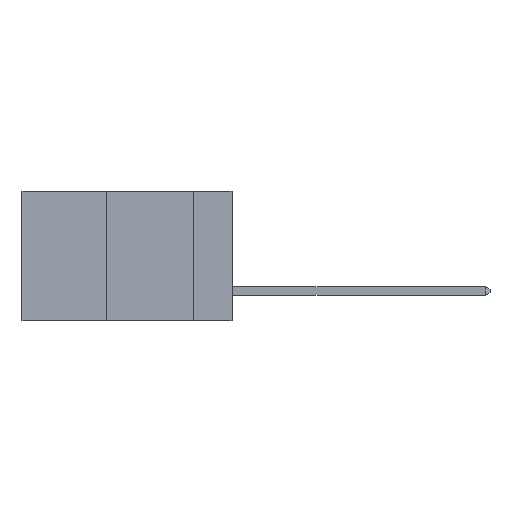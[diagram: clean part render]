
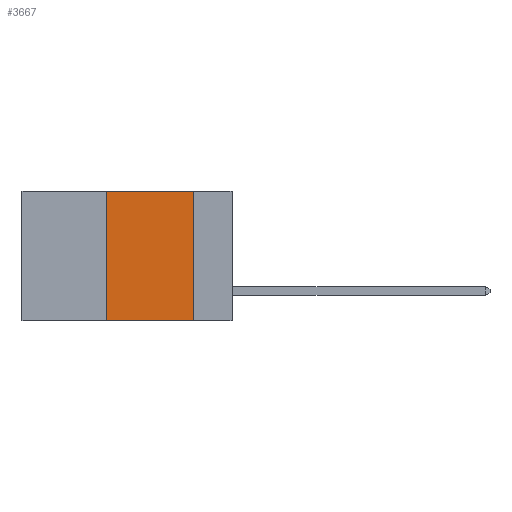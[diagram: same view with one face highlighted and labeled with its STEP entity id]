
A CAD part, left-side view. The second image highlights one B-rep face of the part: STEP entity #3667.
In plain terms, the highlighted planar face has unit normal (-1, 0, 0).
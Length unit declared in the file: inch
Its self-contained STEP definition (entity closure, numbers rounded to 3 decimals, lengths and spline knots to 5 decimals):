
#189 = EDGE_CURVE ( 'NONE', #11978, #1055, #10792, .T. ) ;
#576 = ORIENTED_EDGE ( 'NONE', *, *, #189, .F. ) ;
#738 = CARTESIAN_POINT ( 'NONE',  ( 0., 0.36, 0. ) ) ;
#850 = CARTESIAN_POINT ( 'NONE',  ( 0., 0.6, -0.37 ) ) ;
#1055 = VERTEX_POINT ( 'NONE', #12014 ) ;
#1774 = AXIS2_PLACEMENT_3D ( 'NONE', #11319, #6439, #12218 ) ;
#1845 = DIRECTION ( 'NONE',  ( 0., -1., 0. ) ) ;
#2360 = ORIENTED_EDGE ( 'NONE', *, *, #4052, .F. ) ;
#2379 = CARTESIAN_POINT ( 'NONE',  ( 0., 0.36, -0.37 ) ) ;
#2485 = VERTEX_POINT ( 'NONE', #2379 ) ;
#2753 = CARTESIAN_POINT ( 'NONE',  ( 0., 0.11, 0. ) ) ;
#3005 = DIRECTION ( 'NONE',  ( 0., -1., 0. ) ) ;
#3048 = CARTESIAN_POINT ( 'NONE',  ( 0., 0.6, 0. ) ) ;
#3135 = FACE_OUTER_BOUND ( 'NONE', #11230, .T. ) ;
#3470 = ORIENTED_EDGE ( 'NONE', *, *, #11175, .F. ) ;
#3667 = ADVANCED_FACE ( 'NONE', ( #3135 ), #5649, .F. ) ;
#4052 = EDGE_CURVE ( 'NONE', #4203, #11978, #11677, .T. ) ;
#4203 = VERTEX_POINT ( 'NONE', #738 ) ;
#5649 = PLANE ( 'NONE',  #1774 ) ;
#5791 = LINE ( 'NONE', #6290, #7997 ) ;
#6290 = CARTESIAN_POINT ( 'NONE',  ( 0., 0.36, 0. ) ) ;
#6439 = DIRECTION ( 'NONE',  ( 1., 0., 0. ) ) ;
#7285 = EDGE_CURVE ( 'NONE', #2485, #1055, #7842, .T. ) ;
#7553 = CARTESIAN_POINT ( 'NONE',  ( 0., 0.11, 0. ) ) ;
#7842 = LINE ( 'NONE', #850, #12455 ) ;
#7997 = VECTOR ( 'NONE', #11880, 39.37008 ) ;
#8302 = VECTOR ( 'NONE', #11190, 39.37008 ) ;
#9804 = VECTOR ( 'NONE', #3005, 39.37008 ) ;
#10792 = LINE ( 'NONE', #2753, #8302 ) ;
#11175 = EDGE_CURVE ( 'NONE', #2485, #4203, #5791, .T. ) ;
#11190 = DIRECTION ( 'NONE',  ( 0., 0., -1. ) ) ;
#11230 = EDGE_LOOP ( 'NONE', ( #576, #2360, #3470, #11818 ) ) ;
#11319 = CARTESIAN_POINT ( 'NONE',  ( 0., 0.6, 0. ) ) ;
#11677 = LINE ( 'NONE', #3048, #9804 ) ;
#11818 = ORIENTED_EDGE ( 'NONE', *, *, #7285, .T. ) ;
#11880 = DIRECTION ( 'NONE',  ( 0., 0., 1. ) ) ;
#11978 = VERTEX_POINT ( 'NONE', #7553 ) ;
#12014 = CARTESIAN_POINT ( 'NONE',  ( 0., 0.11, -0.37 ) ) ;
#12218 = DIRECTION ( 'NONE',  ( 0., 0., -1. ) ) ;
#12455 = VECTOR ( 'NONE', #1845, 39.37008 ) ;
